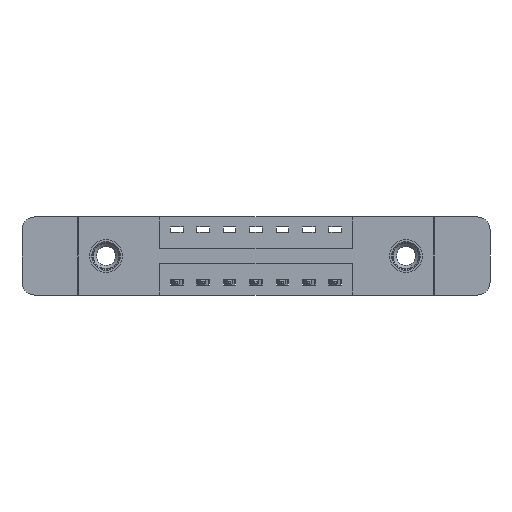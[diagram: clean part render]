
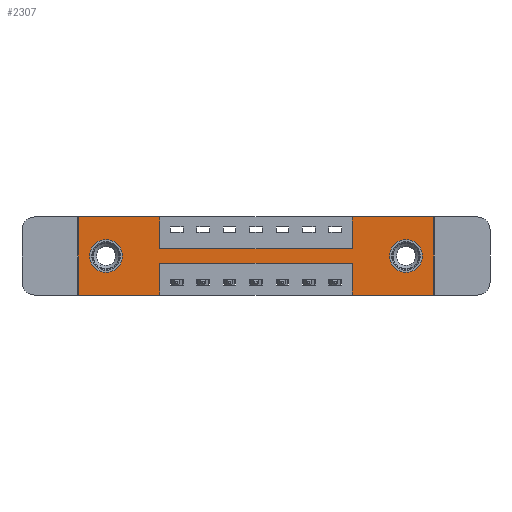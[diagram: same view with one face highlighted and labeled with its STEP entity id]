
A CAD part, front view. The second image highlights one B-rep face of the part: STEP entity #2307.
In plain terms, the highlighted planar face has unit normal (0, -1, 0).
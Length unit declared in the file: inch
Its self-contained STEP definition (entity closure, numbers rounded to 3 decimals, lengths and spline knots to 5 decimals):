
#50 = CARTESIAN_POINT ( 'NONE',  ( 0., 0., -0.37 ) ) ;
#274 = VECTOR ( 'NONE', #6800, 39.37008 ) ;
#496 = EDGE_LOOP ( 'NONE', ( #5844, #3697, #3186, #2385, #10098, #3421, #12159, #1663, #11723, #3418, #12529, #14371 ) ) ;
#524 = CARTESIAN_POINT ( 'NONE',  ( 0., 0., 0. ) ) ;
#589 = VERTEX_POINT ( 'NONE', #1106 ) ;
#630 = VECTOR ( 'NONE', #14615, 39.37008 ) ;
#645 = EDGE_CURVE ( 'NONE', #2258, #5453, #3412, .T. ) ;
#800 = EDGE_CURVE ( 'NONE', #8195, #7523, #2355, .T. ) ;
#841 = DIRECTION ( 'NONE',  ( 1., 0., 0. ) ) ;
#1004 = DIRECTION ( 'NONE',  ( 1., 0., 0. ) ) ;
#1106 = CARTESIAN_POINT ( 'NONE',  ( 1.2975, 0., -0.37 ) ) ;
#1111 = VECTOR ( 'NONE', #1004, 39.37008 ) ;
#1199 = VERTEX_POINT ( 'NONE', #1997 ) ;
#1663 = ORIENTED_EDGE ( 'NONE', *, *, #6278, .F. ) ;
#1719 = LINE ( 'NONE', #5115, #5886 ) ;
#1760 = VECTOR ( 'NONE', #841, 39.37008 ) ;
#1997 = CARTESIAN_POINT ( 'NONE',  ( 0.1325, 0., -0.263 ) ) ;
#2098 = VECTOR ( 'NONE', #2449, 39.37008 ) ;
#2103 = DIRECTION ( 'NONE',  ( 0., 0., 1. ) ) ;
#2258 = VERTEX_POINT ( 'NONE', #5587 ) ;
#2307 = ADVANCED_FACE ( 'NONE', ( #13282, #10199, #4477 ), #8701, .T. ) ;
#2311 = LINE ( 'NONE', #12586, #3960 ) ;
#2355 = LINE ( 'NONE', #6792, #2829 ) ;
#2362 = CARTESIAN_POINT ( 'NONE',  ( 1.2975, 0., -0.15 ) ) ;
#2367 = EDGE_CURVE ( 'NONE', #10674, #5509, #7736, .T. ) ;
#2385 = ORIENTED_EDGE ( 'NONE', *, *, #4511, .F. ) ;
#2449 = DIRECTION ( 'NONE',  ( -1., 0., 0. ) ) ;
#2829 = VECTOR ( 'NONE', #5677, 39.37008 ) ;
#3114 = EDGE_CURVE ( 'NONE', #9856, #6269, #10221, .T. ) ;
#3131 = DIRECTION ( 'NONE',  ( 0., 0., 1. ) ) ;
#3186 = ORIENTED_EDGE ( 'NONE', *, *, #5762, .F. ) ;
#3209 = LINE ( 'NONE', #5435, #1760 ) ;
#3214 = DIRECTION ( 'NONE',  ( 0., 0., -1. ) ) ;
#3245 = VECTOR ( 'NONE', #7870, 39.37008 ) ;
#3299 = CARTESIAN_POINT ( 'NONE',  ( 0.3875, 0., -0.15 ) ) ;
#3362 = DIRECTION ( 'NONE',  ( 0., -1., 0. ) ) ;
#3412 = CIRCLE ( 'NONE', #7432, 0.078 ) ;
#3418 = ORIENTED_EDGE ( 'NONE', *, *, #4982, .F. ) ;
#3421 = ORIENTED_EDGE ( 'NONE', *, *, #14475, .F. ) ;
#3537 = CARTESIAN_POINT ( 'NONE',  ( 0., 0., -0.37 ) ) ;
#3697 = ORIENTED_EDGE ( 'NONE', *, *, #7544, .F. ) ;
#3768 = CARTESIAN_POINT ( 'NONE',  ( 0.3875, 0., -0.22 ) ) ;
#3844 = EDGE_CURVE ( 'NONE', #10282, #9856, #4464, .T. ) ;
#3853 = EDGE_LOOP ( 'NONE', ( #4610, #5585 ) ) ;
#3960 = VECTOR ( 'NONE', #5564, 39.37008 ) ;
#4464 = LINE ( 'NONE', #11240, #3245 ) ;
#4477 = FACE_OUTER_BOUND ( 'NONE', #496, .T. ) ;
#4511 = EDGE_CURVE ( 'NONE', #11116, #589, #9118, .T. ) ;
#4610 = ORIENTED_EDGE ( 'NONE', *, *, #13418, .T. ) ;
#4655 = DIRECTION ( 'NONE',  ( 0., 1., 0. ) ) ;
#4841 = EDGE_CURVE ( 'NONE', #6269, #6932, #1719, .T. ) ;
#4864 = DIRECTION ( 'NONE',  ( 0., 1., 0. ) ) ;
#4932 = DIRECTION ( 'NONE',  ( 0., 0., -1. ) ) ;
#4982 = EDGE_CURVE ( 'NONE', #6932, #8195, #10060, .T. ) ;
#5040 = DIRECTION ( 'NONE',  ( 1., 0., 0. ) ) ;
#5115 = CARTESIAN_POINT ( 'NONE',  ( 0., 0., 0. ) ) ;
#5334 = CARTESIAN_POINT ( 'NONE',  ( 1.2975, 0., -0.22 ) ) ;
#5435 = CARTESIAN_POINT ( 'NONE',  ( 0.3875, 0., -0.15 ) ) ;
#5453 = VERTEX_POINT ( 'NONE', #8232 ) ;
#5463 = AXIS2_PLACEMENT_3D ( 'NONE', #9175, #4655, #6802 ) ;
#5509 = VERTEX_POINT ( 'NONE', #13993 ) ;
#5564 = DIRECTION ( 'NONE',  ( 0., 0., 1. ) ) ;
#5585 = ORIENTED_EDGE ( 'NONE', *, *, #645, .T. ) ;
#5587 = CARTESIAN_POINT ( 'NONE',  ( 1.5525, 0., -0.263 ) ) ;
#5677 = DIRECTION ( 'NONE',  ( 0., 0., -1. ) ) ;
#5762 = EDGE_CURVE ( 'NONE', #589, #13079, #2311, .T. ) ;
#5844 = ORIENTED_EDGE ( 'NONE', *, *, #3844, .F. ) ;
#5886 = VECTOR ( 'NONE', #8526, 39.37008 ) ;
#5896 = LINE ( 'NONE', #13750, #274 ) ;
#6164 = AXIS2_PLACEMENT_3D ( 'NONE', #14226, #11160, #3131 ) ;
#6269 = VERTEX_POINT ( 'NONE', #3537 ) ;
#6278 = EDGE_CURVE ( 'NONE', #7523, #10674, #3209, .T. ) ;
#6478 = CARTESIAN_POINT ( 'NONE',  ( 0., 0., -0.37 ) ) ;
#6682 = CARTESIAN_POINT ( 'NONE',  ( 0., 0., 0. ) ) ;
#6784 = CARTESIAN_POINT ( 'NONE',  ( 0., 0., 0. ) ) ;
#6792 = CARTESIAN_POINT ( 'NONE',  ( 0.3875, 0., 0. ) ) ;
#6800 = DIRECTION ( 'NONE',  ( 0., 0., -1. ) ) ;
#6802 = DIRECTION ( 'NONE',  ( 0., 0., 1. ) ) ;
#6922 = VECTOR ( 'NONE', #11275, 39.37008 ) ;
#6932 = VERTEX_POINT ( 'NONE', #6682 ) ;
#7279 = CARTESIAN_POINT ( 'NONE',  ( 0.3875, 0., -0.37 ) ) ;
#7432 = AXIS2_PLACEMENT_3D ( 'NONE', #8802, #7757, #13167 ) ;
#7523 = VERTEX_POINT ( 'NONE', #3299 ) ;
#7544 = EDGE_CURVE ( 'NONE', #13079, #10282, #12478, .T. ) ;
#7549 = VERTEX_POINT ( 'NONE', #13594 ) ;
#7736 = LINE ( 'NONE', #8928, #9196 ) ;
#7757 = DIRECTION ( 'NONE',  ( 0., 1., 0. ) ) ;
#7818 = CARTESIAN_POINT ( 'NONE',  ( 1.685, 0., 0. ) ) ;
#7870 = DIRECTION ( 'NONE',  ( 0., 0., -1. ) ) ;
#8032 = CARTESIAN_POINT ( 'NONE',  ( 1.685, 0., -0.37 ) ) ;
#8055 = CIRCLE ( 'NONE', #6164, 0.078 ) ;
#8195 = VERTEX_POINT ( 'NONE', #11612 ) ;
#8232 = CARTESIAN_POINT ( 'NONE',  ( 1.5525, 0., -0.107 ) ) ;
#8526 = DIRECTION ( 'NONE',  ( 0., 0., 1. ) ) ;
#8701 = PLANE ( 'NONE',  #13749 ) ;
#8802 = CARTESIAN_POINT ( 'NONE',  ( 1.5525, 0., -0.185 ) ) ;
#8820 = AXIS2_PLACEMENT_3D ( 'NONE', #9168, #4864, #4932 ) ;
#8928 = CARTESIAN_POINT ( 'NONE',  ( 1.2975, 0., 0. ) ) ;
#9118 = LINE ( 'NONE', #11451, #2098 ) ;
#9168 = CARTESIAN_POINT ( 'NONE',  ( 1.5525, 0., -0.185 ) ) ;
#9175 = CARTESIAN_POINT ( 'NONE',  ( 0.1325, 0., -0.185 ) ) ;
#9196 = VECTOR ( 'NONE', #2103, 39.37008 ) ;
#9255 = ORIENTED_EDGE ( 'NONE', *, *, #9561, .T. ) ;
#9321 = VECTOR ( 'NONE', #5040, 39.37008 ) ;
#9561 = EDGE_CURVE ( 'NONE', #1199, #7549, #8055, .T. ) ;
#9856 = VERTEX_POINT ( 'NONE', #7279 ) ;
#10060 = LINE ( 'NONE', #6784, #1111 ) ;
#10098 = ORIENTED_EDGE ( 'NONE', *, *, #10589, .F. ) ;
#10199 = FACE_BOUND ( 'NONE', #14372, .T. ) ;
#10221 = LINE ( 'NONE', #50, #630 ) ;
#10282 = VERTEX_POINT ( 'NONE', #3768 ) ;
#10472 = ORIENTED_EDGE ( 'NONE', *, *, #12062, .T. ) ;
#10589 = EDGE_CURVE ( 'NONE', #11097, #11116, #5896, .T. ) ;
#10674 = VERTEX_POINT ( 'NONE', #2362 ) ;
#10732 = CIRCLE ( 'NONE', #8820, 0.078 ) ;
#10783 = LINE ( 'NONE', #524, #9321 ) ;
#11097 = VERTEX_POINT ( 'NONE', #7818 ) ;
#11116 = VERTEX_POINT ( 'NONE', #8032 ) ;
#11160 = DIRECTION ( 'NONE',  ( 0., 1., 0. ) ) ;
#11240 = CARTESIAN_POINT ( 'NONE',  ( 0.3875, 0., -0.37 ) ) ;
#11275 = DIRECTION ( 'NONE',  ( -1., 0., 0. ) ) ;
#11451 = CARTESIAN_POINT ( 'NONE',  ( 0., 0., -0.37 ) ) ;
#11463 = CIRCLE ( 'NONE', #5463, 0.078 ) ;
#11612 = CARTESIAN_POINT ( 'NONE',  ( 0.3875, 0., 0. ) ) ;
#11723 = ORIENTED_EDGE ( 'NONE', *, *, #800, .F. ) ;
#12062 = EDGE_CURVE ( 'NONE', #7549, #1199, #11463, .T. ) ;
#12159 = ORIENTED_EDGE ( 'NONE', *, *, #2367, .F. ) ;
#12323 = CARTESIAN_POINT ( 'NONE',  ( 0.3875, 0., -0.22 ) ) ;
#12478 = LINE ( 'NONE', #12323, #6922 ) ;
#12529 = ORIENTED_EDGE ( 'NONE', *, *, #4841, .F. ) ;
#12586 = CARTESIAN_POINT ( 'NONE',  ( 1.2975, 0., -0.37 ) ) ;
#13079 = VERTEX_POINT ( 'NONE', #5334 ) ;
#13167 = DIRECTION ( 'NONE',  ( 0., 0., -1. ) ) ;
#13282 = FACE_BOUND ( 'NONE', #3853, .T. ) ;
#13418 = EDGE_CURVE ( 'NONE', #5453, #2258, #10732, .T. ) ;
#13594 = CARTESIAN_POINT ( 'NONE',  ( 0.1325, 0., -0.107 ) ) ;
#13749 = AXIS2_PLACEMENT_3D ( 'NONE', #6478, #3362, #3214 ) ;
#13750 = CARTESIAN_POINT ( 'NONE',  ( 1.685, 0., 0. ) ) ;
#13993 = CARTESIAN_POINT ( 'NONE',  ( 1.2975, 0., 0. ) ) ;
#14226 = CARTESIAN_POINT ( 'NONE',  ( 0.1325, 0., -0.185 ) ) ;
#14371 = ORIENTED_EDGE ( 'NONE', *, *, #3114, .F. ) ;
#14372 = EDGE_LOOP ( 'NONE', ( #10472, #9255 ) ) ;
#14475 = EDGE_CURVE ( 'NONE', #5509, #11097, #10783, .T. ) ;
#14615 = DIRECTION ( 'NONE',  ( -1., 0., 0. ) ) ;
